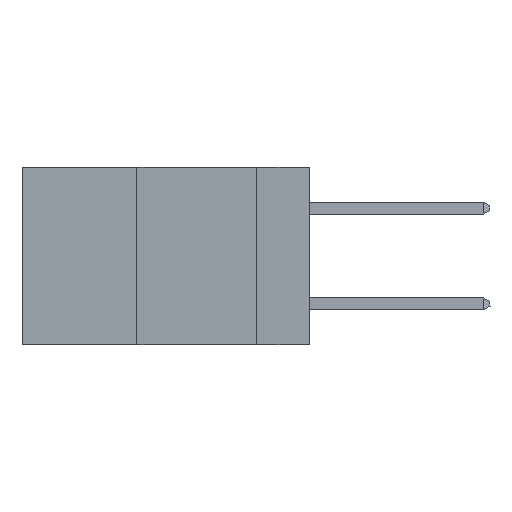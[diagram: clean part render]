
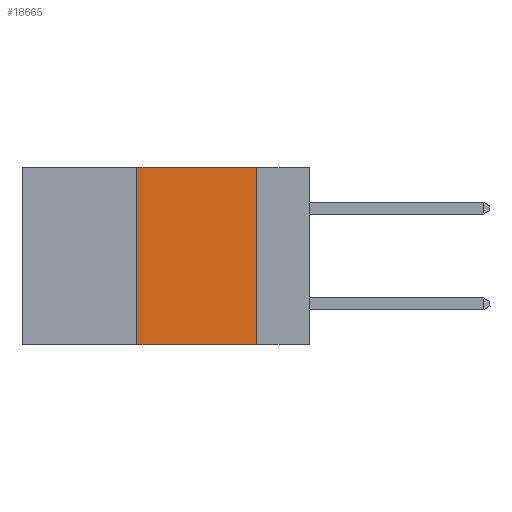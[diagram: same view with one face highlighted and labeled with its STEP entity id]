
A CAD part, left-side view. The second image highlights one B-rep face of the part: STEP entity #18665.
In plain terms, the highlighted planar face has unit normal (-1, 0, 0).
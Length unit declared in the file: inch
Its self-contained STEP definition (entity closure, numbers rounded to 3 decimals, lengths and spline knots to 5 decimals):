
#551 = DIRECTION ( 'NONE',  ( 0., -1., 0. ) ) ;
#2795 = LINE ( 'NONE', #6754, #17470 ) ;
#3269 = ORIENTED_EDGE ( 'NONE', *, *, #14374, .F. ) ;
#3382 = ORIENTED_EDGE ( 'NONE', *, *, #19967, .F. ) ;
#3681 = VERTEX_POINT ( 'NONE', #12140 ) ;
#4335 = VECTOR ( 'NONE', #13123, 39.37008 ) ;
#4877 = CARTESIAN_POINT ( 'NONE',  ( 0., 0.11, 0. ) ) ;
#6349 = LINE ( 'NONE', #22561, #10655 ) ;
#6725 = VERTEX_POINT ( 'NONE', #17342 ) ;
#6754 = CARTESIAN_POINT ( 'NONE',  ( 0., 0.36, 0. ) ) ;
#7263 = VERTEX_POINT ( 'NONE', #20793 ) ;
#8519 = ORIENTED_EDGE ( 'NONE', *, *, #14206, .T. ) ;
#8534 = DIRECTION ( 'NONE',  ( 0., 0., -1. ) ) ;
#8599 = DIRECTION ( 'NONE',  ( 0., 0., 1. ) ) ;
#9518 = VECTOR ( 'NONE', #15811, 39.37008 ) ;
#10308 = PLANE ( 'NONE',  #20797 ) ;
#10655 = VECTOR ( 'NONE', #551, 39.37008 ) ;
#11266 = CARTESIAN_POINT ( 'NONE',  ( 0., 0.6, 0. ) ) ;
#12140 = CARTESIAN_POINT ( 'NONE',  ( 0., 0.36, -0.37 ) ) ;
#13123 = DIRECTION ( 'NONE',  ( 0., -1., 0. ) ) ;
#14206 = EDGE_CURVE ( 'NONE', #3681, #18427, #6349, .T. ) ;
#14354 = LINE ( 'NONE', #4877, #9518 ) ;
#14374 = EDGE_CURVE ( 'NONE', #3681, #7263, #2795, .T. ) ;
#15557 = FACE_OUTER_BOUND ( 'NONE', #17696, .T. ) ;
#15793 = CARTESIAN_POINT ( 'NONE',  ( 0., 0.6, 0. ) ) ;
#15811 = DIRECTION ( 'NONE',  ( 0., 0., -1. ) ) ;
#16995 = CARTESIAN_POINT ( 'NONE',  ( 0., 0.11, -0.37 ) ) ;
#17342 = CARTESIAN_POINT ( 'NONE',  ( 0., 0.11, 0. ) ) ;
#17470 = VECTOR ( 'NONE', #8599, 39.37008 ) ;
#17696 = EDGE_LOOP ( 'NONE', ( #3382, #18432, #3269, #8519 ) ) ;
#18427 = VERTEX_POINT ( 'NONE', #16995 ) ;
#18432 = ORIENTED_EDGE ( 'NONE', *, *, #22536, .F. ) ;
#18665 = ADVANCED_FACE ( 'NONE', ( #15557 ), #10308, .F. ) ;
#18872 = LINE ( 'NONE', #11266, #4335 ) ;
#19413 = DIRECTION ( 'NONE',  ( 1., 0., 0. ) ) ;
#19967 = EDGE_CURVE ( 'NONE', #6725, #18427, #14354, .T. ) ;
#20793 = CARTESIAN_POINT ( 'NONE',  ( 0., 0.36, 0. ) ) ;
#20797 = AXIS2_PLACEMENT_3D ( 'NONE', #15793, #19413, #8534 ) ;
#22536 = EDGE_CURVE ( 'NONE', #7263, #6725, #18872, .T. ) ;
#22561 = CARTESIAN_POINT ( 'NONE',  ( 0., 0.6, -0.37 ) ) ;
